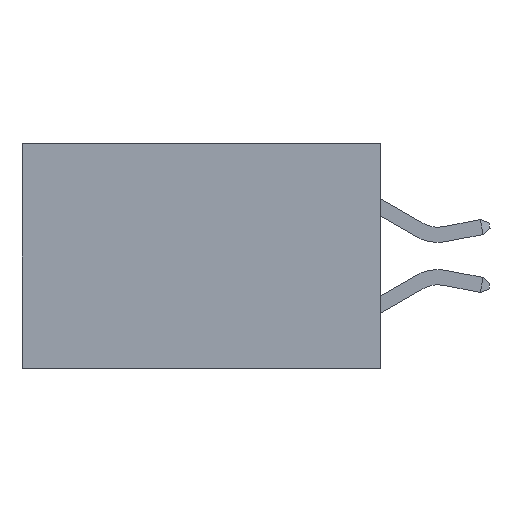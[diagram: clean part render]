
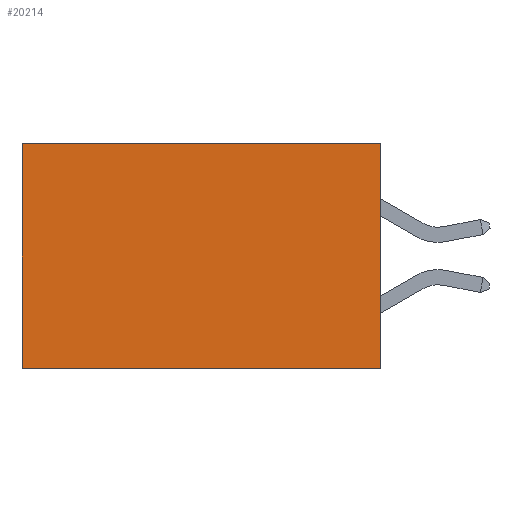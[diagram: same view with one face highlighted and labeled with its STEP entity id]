
A CAD part, left-side view. The second image highlights one B-rep face of the part: STEP entity #20214.
In plain terms, the highlighted planar face has unit normal (-1, 0, 0).
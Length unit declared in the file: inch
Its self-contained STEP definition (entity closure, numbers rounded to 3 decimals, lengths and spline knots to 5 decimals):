
#284 = ORIENTED_EDGE ( 'NONE', *, *, #13616, .F. ) ;
#685 = EDGE_LOOP ( 'NONE', ( #10093, #284, #5489, #1507 ) ) ;
#729 = DIRECTION ( 'NONE',  ( 0., 0., -1. ) ) ;
#1048 = CARTESIAN_POINT ( 'NONE',  ( 0.277, 0.59, 0. ) ) ;
#1507 = ORIENTED_EDGE ( 'NONE', *, *, #20956, .T. ) ;
#2099 = VECTOR ( 'NONE', #23063, 39.37008 ) ;
#2525 = VERTEX_POINT ( 'NONE', #4973 ) ;
#3495 = LINE ( 'NONE', #5487, #14419 ) ;
#4702 = VERTEX_POINT ( 'NONE', #8153 ) ;
#4973 = CARTESIAN_POINT ( 'NONE',  ( 0.277, 0.59, -0.37 ) ) ;
#5343 = LINE ( 'NONE', #11151, #15006 ) ;
#5487 = CARTESIAN_POINT ( 'NONE',  ( 0.277, 0., -0.37 ) ) ;
#5489 = ORIENTED_EDGE ( 'NONE', *, *, #19111, .F. ) ;
#8153 = CARTESIAN_POINT ( 'NONE',  ( 0.277, 0., -0.37 ) ) ;
#10093 = ORIENTED_EDGE ( 'NONE', *, *, #19053, .T. ) ;
#10101 = VERTEX_POINT ( 'NONE', #1048 ) ;
#10435 = CARTESIAN_POINT ( 'NONE',  ( 0.277, 0., 0. ) ) ;
#11151 = CARTESIAN_POINT ( 'NONE',  ( 0.277, 0.59, -0.37 ) ) ;
#11792 = CARTESIAN_POINT ( 'NONE',  ( 0.277, 0., -0.37 ) ) ;
#12419 = DIRECTION ( 'NONE',  ( 1., 0., 0. ) ) ;
#13051 = DIRECTION ( 'NONE',  ( 0., 0., -1. ) ) ;
#13139 = LINE ( 'NONE', #22188, #17530 ) ;
#13616 = EDGE_CURVE ( 'NONE', #4702, #2525, #22522, .T. ) ;
#14060 = FACE_OUTER_BOUND ( 'NONE', #685, .T. ) ;
#14419 = VECTOR ( 'NONE', #18892, 39.37008 ) ;
#15006 = VECTOR ( 'NONE', #13051, 39.37008 ) ;
#15338 = AXIS2_PLACEMENT_3D ( 'NONE', #23680, #12419, #729 ) ;
#17530 = VECTOR ( 'NONE', #24093, 39.37008 ) ;
#18892 = DIRECTION ( 'NONE',  ( 0., 0., -1. ) ) ;
#19053 = EDGE_CURVE ( 'NONE', #10101, #2525, #5343, .T. ) ;
#19111 = EDGE_CURVE ( 'NONE', #19476, #4702, #3495, .T. ) ;
#19476 = VERTEX_POINT ( 'NONE', #10435 ) ;
#19909 = PLANE ( 'NONE',  #15338 ) ;
#20214 = ADVANCED_FACE ( 'NONE', ( #14060 ), #19909, .F. ) ;
#20956 = EDGE_CURVE ( 'NONE', #19476, #10101, #13139, .T. ) ;
#22188 = CARTESIAN_POINT ( 'NONE',  ( 0.277, 0., 0. ) ) ;
#22522 = LINE ( 'NONE', #11792, #2099 ) ;
#23063 = DIRECTION ( 'NONE',  ( 0., 1., 0. ) ) ;
#23680 = CARTESIAN_POINT ( 'NONE',  ( 0.277, 0., -0.37 ) ) ;
#24093 = DIRECTION ( 'NONE',  ( 0., 1., 0. ) ) ;
